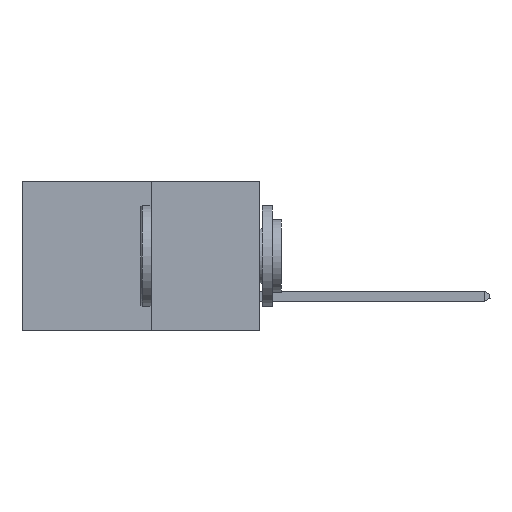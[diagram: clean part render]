
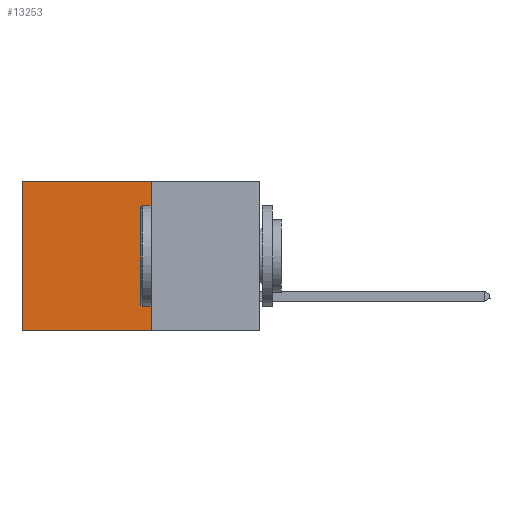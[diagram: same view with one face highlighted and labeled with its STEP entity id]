
A CAD part, left-side view. The second image highlights one B-rep face of the part: STEP entity #13253.
In plain terms, the highlighted planar face has unit normal (-1, 0, 0).
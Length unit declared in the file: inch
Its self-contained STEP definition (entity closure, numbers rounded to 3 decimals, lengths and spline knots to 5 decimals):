
#482 = AXIS2_PLACEMENT_3D ( 'NONE', #2707, #14283, #6671 ) ;
#1477 = CARTESIAN_POINT ( 'NONE',  ( 0.277, 0.59, -0.37 ) ) ;
#1699 = LINE ( 'NONE', #15504, #4344 ) ;
#1919 = CARTESIAN_POINT ( 'NONE',  ( 0.277, 0.27, 0. ) ) ;
#2040 = ORIENTED_EDGE ( 'NONE', *, *, #10974, .T. ) ;
#2707 = CARTESIAN_POINT ( 'NONE',  ( 0.277, 0.27, -0.37 ) ) ;
#2763 = VECTOR ( 'NONE', #3792, 39.37008 ) ;
#3048 = VERTEX_POINT ( 'NONE', #1477 ) ;
#3582 = DIRECTION ( 'NONE',  ( 0., 0., -1. ) ) ;
#3610 = CARTESIAN_POINT ( 'NONE',  ( 0.277, 0.27, -0.37 ) ) ;
#3792 = DIRECTION ( 'NONE',  ( 0., 1., 0. ) ) ;
#4344 = VECTOR ( 'NONE', #11799, 39.37008 ) ;
#5330 = PLANE ( 'NONE',  #482 ) ;
#5486 = CARTESIAN_POINT ( 'NONE',  ( 0.277, 0.27, -0.37 ) ) ;
#5882 = VERTEX_POINT ( 'NONE', #1919 ) ;
#5904 = ORIENTED_EDGE ( 'NONE', *, *, #8690, .F. ) ;
#6296 = EDGE_CURVE ( 'NONE', #5882, #13988, #14181, .T. ) ;
#6573 = CARTESIAN_POINT ( 'NONE',  ( 0.277, 0.27, -0.37 ) ) ;
#6644 = DIRECTION ( 'NONE',  ( 0., 0., -1. ) ) ;
#6671 = DIRECTION ( 'NONE',  ( 0., 0., -1. ) ) ;
#7812 = FACE_OUTER_BOUND ( 'NONE', #11286, .T. ) ;
#7817 = VECTOR ( 'NONE', #6644, 39.37008 ) ;
#8391 = LINE ( 'NONE', #8712, #14727 ) ;
#8690 = EDGE_CURVE ( 'NONE', #13988, #3048, #9275, .T. ) ;
#8712 = CARTESIAN_POINT ( 'NONE',  ( 0.277, 0.59, -0.37 ) ) ;
#9275 = LINE ( 'NONE', #3610, #2763 ) ;
#10974 = EDGE_CURVE ( 'NONE', #5882, #12782, #1699, .T. ) ;
#11286 = EDGE_LOOP ( 'NONE', ( #15623, #5904, #16580, #2040 ) ) ;
#11464 = CARTESIAN_POINT ( 'NONE',  ( 0.277, 0.59, 0. ) ) ;
#11799 = DIRECTION ( 'NONE',  ( 0., 1., 0. ) ) ;
#12048 = EDGE_CURVE ( 'NONE', #12782, #3048, #8391, .T. ) ;
#12782 = VERTEX_POINT ( 'NONE', #11464 ) ;
#13253 = ADVANCED_FACE ( 'NONE', ( #7812 ), #5330, .F. ) ;
#13988 = VERTEX_POINT ( 'NONE', #5486 ) ;
#14181 = LINE ( 'NONE', #6573, #7817 ) ;
#14283 = DIRECTION ( 'NONE',  ( 1., 0., 0. ) ) ;
#14727 = VECTOR ( 'NONE', #3582, 39.37008 ) ;
#15504 = CARTESIAN_POINT ( 'NONE',  ( 0.277, 0.27, 0. ) ) ;
#15623 = ORIENTED_EDGE ( 'NONE', *, *, #12048, .T. ) ;
#16580 = ORIENTED_EDGE ( 'NONE', *, *, #6296, .F. ) ;
